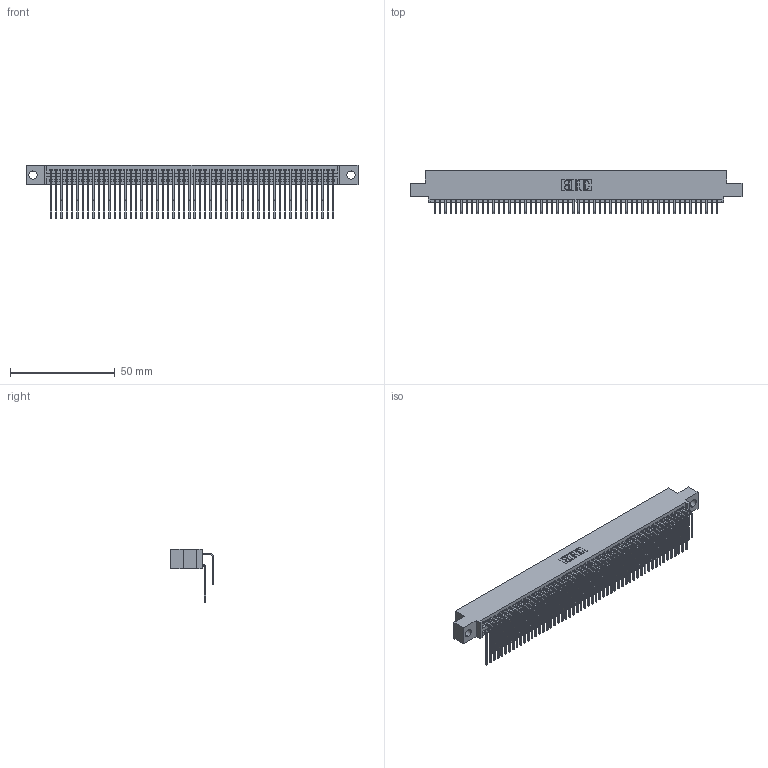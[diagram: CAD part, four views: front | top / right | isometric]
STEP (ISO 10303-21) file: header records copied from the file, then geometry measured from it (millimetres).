
FILE_DESCRIPTION (( 'STEP AP203' ), '1' );
FILE_NAME ('395-108-559-504.STEP', '2018-12-01T00:24:56', ( '' ), ( '' ), 'SwSTEP 2.0', 'SolidWorks 2016', '' );
FILE_SCHEMA (( 'CONFIG_CONTROL_DESIGN' ));
Length unit declared in the file: inch
Products named in the file (4): 345-292-001_559 Tail - 2; 345-292-001_558 559 Tail - 1; 345 Part_0.110 Offset - 0.156 Dia-TH; 395-108-559-504
Assembly tree (109 placements, depth 2):
  395-108-559-504
    345 Part_0.110 Offset - 0.156 Dia-TH
    345-292-001_558 559 Tail - 1  x54
    345-292-001_559 Tail - 2  x54
Bounding box: 158.37 x 20.56 x 25.53 mm (x, y, z)
Volume: 15957.3 mm3; surface area: 26657.7 mm2
Topology: 109 solids, 109 shells, 5746 faces, 17093 edges, 11250 vertices
Faces by surface type: plane 3864, cylinder 1882
Entity records: 42541 total; most frequent: CARTESIAN_POINT 7167, ORIENTED_EDGE 7050, DIRECTION 6277, EDGE_CURVE 3525, LINE 3137, VECTOR 3137, VERTEX_POINT 2346, AXIS2_PLACEMENT_3D 1570
